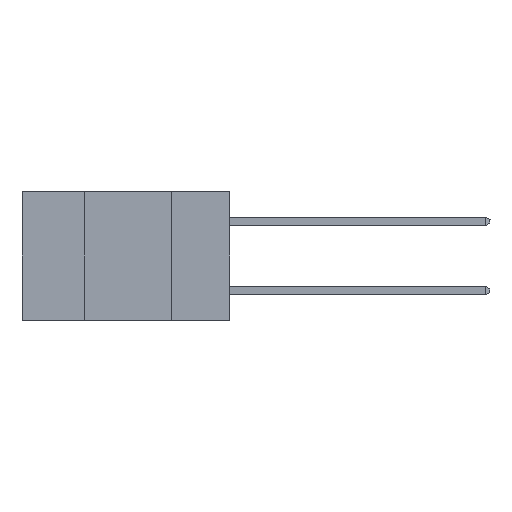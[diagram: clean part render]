
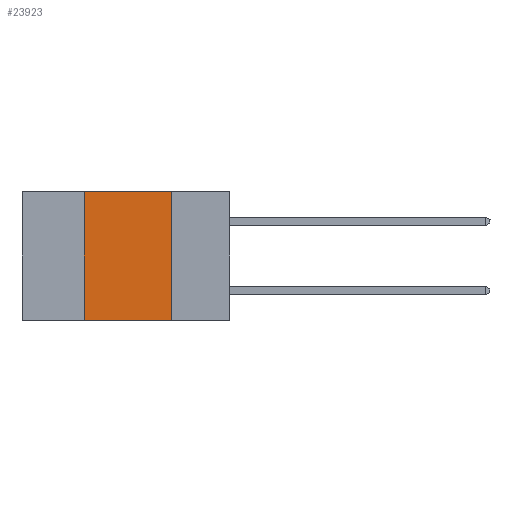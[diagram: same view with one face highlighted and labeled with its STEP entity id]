
A CAD part, left-side view. The second image highlights one B-rep face of the part: STEP entity #23923.
In plain terms, the highlighted planar face has unit normal (-1, 0, 0).
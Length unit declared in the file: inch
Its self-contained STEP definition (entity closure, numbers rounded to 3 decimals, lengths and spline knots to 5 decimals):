
#635 = EDGE_CURVE ( 'NONE', #5394, #21448, #4803, .T. ) ;
#769 = CARTESIAN_POINT ( 'NONE',  ( 0., 0.17, -0.37 ) ) ;
#888 = DIRECTION ( 'NONE',  ( 0., 0., 1. ) ) ;
#1016 = LINE ( 'NONE', #769, #19728 ) ;
#1068 = DIRECTION ( 'NONE',  ( 0., -1., 0. ) ) ;
#1523 = EDGE_CURVE ( 'NONE', #9176, #21593, #23517, .T. ) ;
#2296 = DIRECTION ( 'NONE',  ( 1., 0., 0. ) ) ;
#3631 = EDGE_LOOP ( 'NONE', ( #19737, #16721, #17775, #8124 ) ) ;
#3912 = FACE_OUTER_BOUND ( 'NONE', #3631, .T. ) ;
#4061 = VECTOR ( 'NONE', #888, 39.37008 ) ;
#4295 = CARTESIAN_POINT ( 'NONE',  ( 0., 0.42, 0. ) ) ;
#4635 = LINE ( 'NONE', #13744, #4061 ) ;
#4803 = LINE ( 'NONE', #21771, #19834 ) ;
#5394 = VERTEX_POINT ( 'NONE', #17230 ) ;
#7662 = CARTESIAN_POINT ( 'NONE',  ( 0., 0.6, 0. ) ) ;
#8124 = ORIENTED_EDGE ( 'NONE', *, *, #635, .T. ) ;
#8776 = DIRECTION ( 'NONE',  ( 0., -1., 0. ) ) ;
#9176 = VERTEX_POINT ( 'NONE', #4295 ) ;
#11943 = CARTESIAN_POINT ( 'NONE',  ( 0., 0.17, -0.37 ) ) ;
#12609 = DIRECTION ( 'NONE',  ( 0., 0., -1. ) ) ;
#13744 = CARTESIAN_POINT ( 'NONE',  ( 0., 0.42, -0.37 ) ) ;
#14415 = EDGE_CURVE ( 'NONE', #5394, #9176, #4635, .T. ) ;
#14647 = AXIS2_PLACEMENT_3D ( 'NONE', #7662, #2296, #15285 ) ;
#15285 = DIRECTION ( 'NONE',  ( 0., 0., -1. ) ) ;
#16721 = ORIENTED_EDGE ( 'NONE', *, *, #1523, .F. ) ;
#17230 = CARTESIAN_POINT ( 'NONE',  ( 0., 0.42, -0.37 ) ) ;
#17775 = ORIENTED_EDGE ( 'NONE', *, *, #14415, .F. ) ;
#19224 = VECTOR ( 'NONE', #8776, 39.37008 ) ;
#19405 = PLANE ( 'NONE',  #14647 ) ;
#19728 = VECTOR ( 'NONE', #12609, 39.37008 ) ;
#19737 = ORIENTED_EDGE ( 'NONE', *, *, #20522, .F. ) ;
#19782 = CARTESIAN_POINT ( 'NONE',  ( 0., 0.6, 0. ) ) ;
#19834 = VECTOR ( 'NONE', #1068, 39.37008 ) ;
#20522 = EDGE_CURVE ( 'NONE', #21593, #21448, #1016, .T. ) ;
#21448 = VERTEX_POINT ( 'NONE', #11943 ) ;
#21593 = VERTEX_POINT ( 'NONE', #22529 ) ;
#21771 = CARTESIAN_POINT ( 'NONE',  ( 0., 0.6, -0.37 ) ) ;
#22529 = CARTESIAN_POINT ( 'NONE',  ( 0., 0.17, 0. ) ) ;
#23517 = LINE ( 'NONE', #19782, #19224 ) ;
#23923 = ADVANCED_FACE ( 'NONE', ( #3912 ), #19405, .F. ) ;
